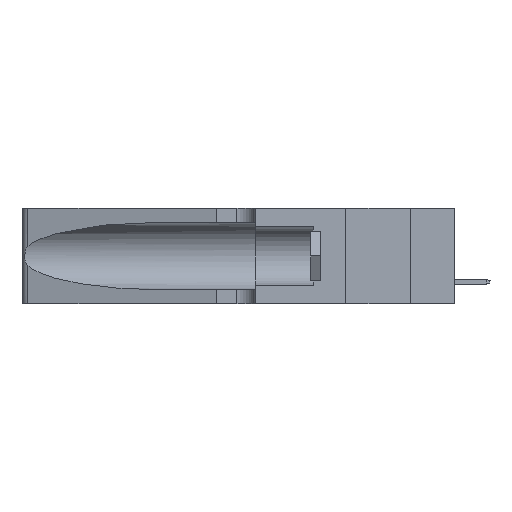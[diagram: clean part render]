
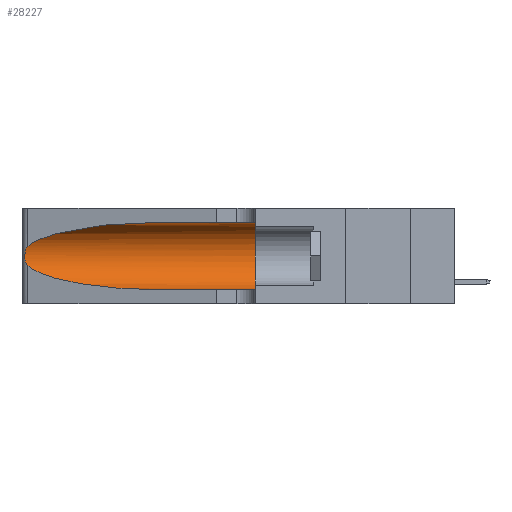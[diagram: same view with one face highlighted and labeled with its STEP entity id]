
A CAD part, left-side view. The second image highlights one B-rep face of the part: STEP entity #28227.
In plain terms, the highlighted cylindrical face has radius 3.308 mm (diameter 6.617 mm), a partial arc.
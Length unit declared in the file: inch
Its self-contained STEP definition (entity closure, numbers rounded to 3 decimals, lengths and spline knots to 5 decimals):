
#2540 = CARTESIAN_POINT ( 'NONE',  ( 0.1305, 1.61858, 0.31525 ) ) ;
#2548 = ORIENTED_EDGE ( 'NONE', *, *, #11347, .F. ) ;
#2737 = CARTESIAN_POINT ( 'NONE',  ( 0.1305, 0.35, 0.31525 ) ) ;
#3667 = CARTESIAN_POINT ( 'NONE',  ( 0.25555, 1.22994, 0.2215 ) ) ;
#4176 = EDGE_CURVE ( 'NONE', #20693, #30061, #21939, .T. ) ;
#4800 = CYLINDRICAL_SURFACE ( 'NONE', #16124, 0.13025 ) ;
#5608 = CARTESIAN_POINT ( 'NONE',  ( 0.1305, 1.61858, 0.185 ) ) ;
#5701 = CARTESIAN_POINT ( 'NONE',  ( 0.1305, 0.72297, 0.31525 ) ) ;
#6156 = CARTESIAN_POINT ( 'NONE',  ( 0.25639, 1.23186, 0.15144 ) ) ;
#6554 = CARTESIAN_POINT ( 'NONE',  ( 0.25487, 1.22718, 0.14631 ) ) ;
#6890 = EDGE_CURVE ( 'NONE', #10590, #10242, #35085, .T. ) ;
#8071 = VERTEX_POINT ( 'NONE', #2737 ) ;
#8491 = CARTESIAN_POINT ( 'NONE',  ( 0.1305, 0.72297, 0.31525 ) ) ;
#10242 = VERTEX_POINT ( 'NONE', #6554 ) ;
#10590 = VERTEX_POINT ( 'NONE', #24645 ) ;
#10888 = CARTESIAN_POINT ( 'NONE',  ( 0.2373, 1.15595, 0.08982 ) ) ;
#11347 = EDGE_CURVE ( 'NONE', #27282, #8071, #12455, .T. ) ;
#11924 = ORIENTED_EDGE ( 'NONE', *, *, #4176, .T. ) ;
#12377 = CARTESIAN_POINT ( 'NONE',  ( 0.1305, 0.35, 0.05475 ) ) ;
#12455 = LINE ( 'NONE', #2540, #12742 ) ;
#12548 = CARTESIAN_POINT ( 'NONE',  ( 0.26075, 1.23896, 0.19203 ) ) ;
#12742 = VECTOR ( 'NONE', #28308, 39.37008 ) ;
#13670 = CARTESIAN_POINT ( 'NONE',  ( 0.1305, 0.35, 0.185 ) ) ;
#13777 = CARTESIAN_POINT ( 'NONE',  ( 0.18966, 0.96281, 0.05475 ) ) ;
#14456 = DIRECTION ( 'NONE',  ( 0., 0., 1. ) ) ;
#14674 = CARTESIAN_POINT ( 'NONE',  ( 0.18966, 0.96281, 0.31525 ) ) ;
#15159 = CARTESIAN_POINT ( 'NONE',  ( 0.1305, 1.61858, 0.05475 ) ) ;
#16124 = AXIS2_PLACEMENT_3D ( 'NONE', #5608, #27227, #33639 ) ;
#16248 = CARTESIAN_POINT ( 'NONE',  ( 0.25639, 1.23184, 0.21858 ) ) ;
#16957 = DIRECTION ( 'NONE',  ( 0., 1., 0. ) ) ;
#17569 = CARTESIAN_POINT ( 'NONE',  ( 0.2373, 1.15595, 0.28018 ) ) ;
#17643 = ORIENTED_EDGE ( 'NONE', *, *, #6890, .T. ) ;
#18566 = ORIENTED_EDGE ( 'NONE', *, *, #37040, .T. ) ;
#19114 = CARTESIAN_POINT ( 'NONE',  ( 0.25854, 1.2359, 0.20912 ) ) ;
#20693 = VERTEX_POINT ( 'NONE', #35803 ) ;
#21939 = LINE ( 'NONE', #15159, #24686 ) ;
#23249 = CIRCLE ( 'NONE', #26548, 0.13025 ) ;
#23822 = CARTESIAN_POINT ( 'NONE',  ( 0.25487, 1.22718, 0.14631 ) ) ;
#24645 = CARTESIAN_POINT ( 'NONE',  ( 0.25487, 1.22718, 0.22369 ) ) ;
#24686 = VECTOR ( 'NONE', #27930, 39.37008 ) ;
#25291 = CARTESIAN_POINT ( 'NONE',  ( 0.26075, 1.23896, 0.178 ) ) ;
#25697 = CARTESIAN_POINT ( 'NONE',  ( 0.25789, 1.23486, 0.15765 ) ) ;
#26548 = AXIS2_PLACEMENT_3D ( 'NONE', #13670, #16957, #14456 ) ;
#26731 = CARTESIAN_POINT ( 'NONE',  ( 0.1305, 0.72297, 0.05475 ) ) ;
#26784 = EDGE_CURVE ( 'NONE', #8071, #30061, #23249, .T. ) ;
#27227 = DIRECTION ( 'NONE',  ( 0., -1., 0. ) ) ;
#27282 = VERTEX_POINT ( 'NONE', #5701 ) ;
#27930 = DIRECTION ( 'NONE',  ( 0., -1., 0. ) ) ;
#28227 = ADVANCED_FACE ( 'NONE', ( #30331 ), #4800, .F. ) ;
#28308 = DIRECTION ( 'NONE',  ( 0., -1., 0. ) ) ;
#28604 = CARTESIAN_POINT ( 'NONE',  ( 0.25487, 1.22718, 0.14631 ) ) ;
#29165 = EDGE_LOOP ( 'NONE', ( #18566, #17643, #36709, #11924, #38029, #2548 ) ) ;
#30061 = VERTEX_POINT ( 'NONE', #12377 ) ;
#30331 = FACE_OUTER_BOUND ( 'NONE', #29165, .T. ) ;
#31141 =( BOUNDED_CURVE ( )  B_SPLINE_CURVE ( 3, ( #8491, #14674, #17569, #39267 ),
 .UNSPECIFIED., .F., .F. ) 
 B_SPLINE_CURVE_WITH_KNOTS ( ( 4, 4 ),
 ( 1.5708, 2.84003 ),
 .UNSPECIFIED. ) 
 CURVE ( )  GEOMETRIC_REPRESENTATION_ITEM ( )  RATIONAL_B_SPLINE_CURVE ( ( 1., 0.87, 0.87, 1. ) ) 
 REPRESENTATION_ITEM ( '' )  );
#31311 = CARTESIAN_POINT ( 'NONE',  ( 0.25555, 1.22993, 0.14849 ) ) ;
#31700 = CARTESIAN_POINT ( 'NONE',  ( 0.26017, 1.23833, 0.17102 ) ) ;
#31776 = EDGE_CURVE ( 'NONE', #10242, #20693, #36917, .T. ) ;
#31907 = CARTESIAN_POINT ( 'NONE',  ( 0.25487, 1.22718, 0.22369 ) ) ;
#33639 = DIRECTION ( 'NONE',  ( 0., 0., -1. ) ) ;
#34612 = CARTESIAN_POINT ( 'NONE',  ( 0.25787, 1.23484, 0.2124 ) ) ;
#35085 = B_SPLINE_CURVE_WITH_KNOTS ( 'NONE', 3,
 ( #31907, #3667, #16248, #34612, #19114, #36643, #12548, #25291, #31700, #37920, #25697, #6156, #31311, #28604 ),
 .UNSPECIFIED., .F., .F.,
 ( 4, 2, 2, 2, 2, 2, 4 ),
 ( 0., 0.00027, 0.00053, 0.00107, 0.0016, 0.00187, 0.00214 ),
 .UNSPECIFIED. ) ;
#35803 = CARTESIAN_POINT ( 'NONE',  ( 0.1305, 0.72297, 0.05475 ) ) ;
#36643 = CARTESIAN_POINT ( 'NONE',  ( 0.26018, 1.23835, 0.19895 ) ) ;
#36709 = ORIENTED_EDGE ( 'NONE', *, *, #31776, .T. ) ;
#36917 =( BOUNDED_CURVE ( )  B_SPLINE_CURVE ( 3, ( #23822, #10888, #13777, #26731 ),
 .UNSPECIFIED., .F., .T. ) 
 B_SPLINE_CURVE_WITH_KNOTS ( ( 4, 4 ),
 ( 3.44316, 4.71239 ),
 .UNSPECIFIED. ) 
 CURVE ( )  GEOMETRIC_REPRESENTATION_ITEM ( )  RATIONAL_B_SPLINE_CURVE ( ( 1., 0.87, 0.87, 1. ) ) 
 REPRESENTATION_ITEM ( '' )  );
#37040 = EDGE_CURVE ( 'NONE', #27282, #10590, #31141, .T. ) ;
#37920 = CARTESIAN_POINT ( 'NONE',  ( 0.25856, 1.23593, 0.16098 ) ) ;
#38029 = ORIENTED_EDGE ( 'NONE', *, *, #26784, .F. ) ;
#39267 = CARTESIAN_POINT ( 'NONE',  ( 0.25487, 1.22718, 0.22369 ) ) ;
